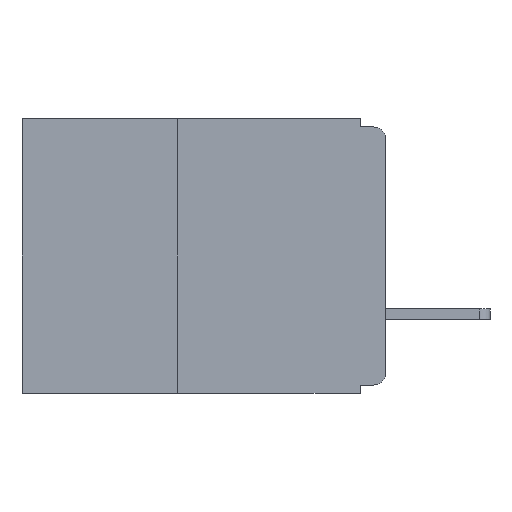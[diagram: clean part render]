
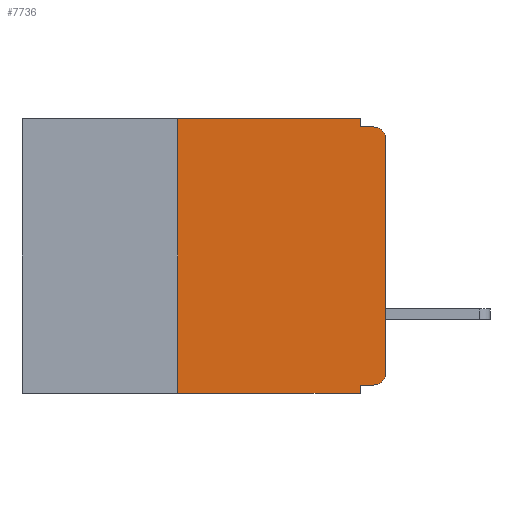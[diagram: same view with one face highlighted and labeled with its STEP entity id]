
A CAD part, left-side view. The second image highlights one B-rep face of the part: STEP entity #7736.
In plain terms, the highlighted planar face has unit normal (-1, 0, 0).
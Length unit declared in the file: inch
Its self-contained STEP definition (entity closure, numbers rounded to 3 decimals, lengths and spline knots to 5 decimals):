
#36 = CARTESIAN_POINT ( 'NONE',  ( 0., 0.015, -0.025 ) ) ;
#350 = VECTOR ( 'NONE', #7086, 39.37008 ) ;
#393 = DIRECTION ( 'NONE',  ( 0., 0., -1. ) ) ;
#463 = EDGE_CURVE ( 'NONE', #11150, #12889, #9866, .T. ) ;
#574 = VECTOR ( 'NONE', #9082, 39.37008 ) ;
#981 = DIRECTION ( 'NONE',  ( 0., -1., 0. ) ) ;
#1193 = VERTEX_POINT ( 'NONE', #3735 ) ;
#1341 = LINE ( 'NONE', #7825, #574 ) ;
#1490 = AXIS2_PLACEMENT_3D ( 'NONE', #36, #14864, #14790 ) ;
#2018 = DIRECTION ( 'NONE',  ( 0., -1., 0. ) ) ;
#2268 = EDGE_CURVE ( 'NONE', #13959, #12069, #10778, .T. ) ;
#2295 = VECTOR ( 'NONE', #981, 39.37008 ) ;
#2307 = EDGE_CURVE ( 'NONE', #7381, #14250, #1341, .T. ) ;
#2364 = EDGE_CURVE ( 'NONE', #7381, #10850, #9345, .T. ) ;
#2382 = EDGE_CURVE ( 'NONE', #1193, #10850, #6966, .T. ) ;
#2611 = DIRECTION ( 'NONE',  ( 1., 0., 0. ) ) ;
#2643 = VECTOR ( 'NONE', #8469, 39.37008 ) ;
#2658 = FACE_OUTER_BOUND ( 'NONE', #6502, .T. ) ;
#3180 = CARTESIAN_POINT ( 'NONE',  ( 0., 0., 0. ) ) ;
#3187 = EDGE_CURVE ( 'NONE', #3240, #11150, #5830, .T. ) ;
#3240 = VERTEX_POINT ( 'NONE', #9388 ) ;
#3735 = CARTESIAN_POINT ( 'NONE',  ( 0., 0.031, -0.32 ) ) ;
#4270 = CARTESIAN_POINT ( 'NONE',  ( 0., 0.031, -0.33 ) ) ;
#5061 = PLANE ( 'NONE',  #8409 ) ;
#5170 = EDGE_CURVE ( 'NONE', #12889, #7008, #13289, .T. ) ;
#5210 = AXIS2_PLACEMENT_3D ( 'NONE', #14154, #14049, #393 ) ;
#5291 = LINE ( 'NONE', #5595, #13723 ) ;
#5462 = ORIENTED_EDGE ( 'NONE', *, *, #3187, .T. ) ;
#5595 = CARTESIAN_POINT ( 'NONE',  ( 0., 0.437, 0. ) ) ;
#5629 = DIRECTION ( 'NONE',  ( 0., 0., -1. ) ) ;
#5720 = CARTESIAN_POINT ( 'NONE',  ( 0., 0.25, -0.33 ) ) ;
#5830 = CIRCLE ( 'NONE', #5210, 0.015 ) ;
#5938 = EDGE_CURVE ( 'NONE', #3240, #1193, #8191, .T. ) ;
#6207 = VECTOR ( 'NONE', #6438, 39.37008 ) ;
#6230 = CARTESIAN_POINT ( 'NONE',  ( 0., 0.031, -0.01 ) ) ;
#6387 = CARTESIAN_POINT ( 'NONE',  ( 0., 0.437, -0.33 ) ) ;
#6438 = DIRECTION ( 'NONE',  ( 0., -1., 0. ) ) ;
#6502 = EDGE_LOOP ( 'NONE', ( #10308, #10678, #10738, #10979, #11103, #11170, #11186, #12161, #13504, #5462 ) ) ;
#6610 = CARTESIAN_POINT ( 'NONE',  ( 0., 0., -0.025 ) ) ;
#6671 = CARTESIAN_POINT ( 'NONE',  ( 0., 0.031, -0.33 ) ) ;
#6966 = LINE ( 'NONE', #6671, #2643 ) ;
#7008 = VERTEX_POINT ( 'NONE', #12957 ) ;
#7086 = DIRECTION ( 'NONE',  ( 0., 0., 1. ) ) ;
#7381 = VERTEX_POINT ( 'NONE', #5720 ) ;
#7736 = ADVANCED_FACE ( 'NONE', ( #2658 ), #5061, .F. ) ;
#7825 = CARTESIAN_POINT ( 'NONE',  ( 0., 0.25, -0.33 ) ) ;
#8191 = LINE ( 'NONE', #11132, #10858 ) ;
#8409 = AXIS2_PLACEMENT_3D ( 'NONE', #12268, #2611, #5629 ) ;
#8469 = DIRECTION ( 'NONE',  ( 0., 0., -1. ) ) ;
#8715 = DIRECTION ( 'NONE',  ( 0., 0., -1. ) ) ;
#9007 = LINE ( 'NONE', #9276, #2295 ) ;
#9082 = DIRECTION ( 'NONE',  ( 0., 0., 1. ) ) ;
#9241 = CARTESIAN_POINT ( 'NONE',  ( 0., 0.031, 0. ) ) ;
#9276 = CARTESIAN_POINT ( 'NONE',  ( 0., 0., -0.01 ) ) ;
#9345 = LINE ( 'NONE', #6387, #6207 ) ;
#9388 = CARTESIAN_POINT ( 'NONE',  ( 0., 0.015, -0.32 ) ) ;
#9866 = LINE ( 'NONE', #3180, #350 ) ;
#10245 = DIRECTION ( 'NONE',  ( 0., 1., 0. ) ) ;
#10308 = ORIENTED_EDGE ( 'NONE', *, *, #463, .T. ) ;
#10678 = ORIENTED_EDGE ( 'NONE', *, *, #5170, .T. ) ;
#10738 = ORIENTED_EDGE ( 'NONE', *, *, #14327, .F. ) ;
#10778 = LINE ( 'NONE', #9241, #13732 ) ;
#10850 = VERTEX_POINT ( 'NONE', #4270 ) ;
#10858 = VECTOR ( 'NONE', #10245, 39.37008 ) ;
#10979 = ORIENTED_EDGE ( 'NONE', *, *, #2268, .F. ) ;
#11103 = ORIENTED_EDGE ( 'NONE', *, *, #14733, .F. ) ;
#11132 = CARTESIAN_POINT ( 'NONE',  ( 0., 0., -0.32 ) ) ;
#11150 = VERTEX_POINT ( 'NONE', #12951 ) ;
#11170 = ORIENTED_EDGE ( 'NONE', *, *, #2307, .F. ) ;
#11186 = ORIENTED_EDGE ( 'NONE', *, *, #2364, .T. ) ;
#11958 = CARTESIAN_POINT ( 'NONE',  ( 0., 0.031, 0. ) ) ;
#12069 = VERTEX_POINT ( 'NONE', #6230 ) ;
#12161 = ORIENTED_EDGE ( 'NONE', *, *, #2382, .F. ) ;
#12268 = CARTESIAN_POINT ( 'NONE',  ( 0., 0.437, 0. ) ) ;
#12889 = VERTEX_POINT ( 'NONE', #6610 ) ;
#12951 = CARTESIAN_POINT ( 'NONE',  ( 0., 0., -0.305 ) ) ;
#12957 = CARTESIAN_POINT ( 'NONE',  ( 0., 0.015, -0.01 ) ) ;
#13289 = CIRCLE ( 'NONE', #1490, 0.015 ) ;
#13504 = ORIENTED_EDGE ( 'NONE', *, *, #5938, .F. ) ;
#13636 = CARTESIAN_POINT ( 'NONE',  ( 0., 0.25, 0. ) ) ;
#13723 = VECTOR ( 'NONE', #2018, 39.37008 ) ;
#13732 = VECTOR ( 'NONE', #8715, 39.37008 ) ;
#13959 = VERTEX_POINT ( 'NONE', #11958 ) ;
#14049 = DIRECTION ( 'NONE',  ( -1., 0., 0. ) ) ;
#14154 = CARTESIAN_POINT ( 'NONE',  ( 0., 0.015, -0.305 ) ) ;
#14250 = VERTEX_POINT ( 'NONE', #13636 ) ;
#14327 = EDGE_CURVE ( 'NONE', #12069, #7008, #9007, .T. ) ;
#14733 = EDGE_CURVE ( 'NONE', #14250, #13959, #5291, .T. ) ;
#14790 = DIRECTION ( 'NONE',  ( 0., 0., -1. ) ) ;
#14864 = DIRECTION ( 'NONE',  ( -1., 0., 0. ) ) ;
